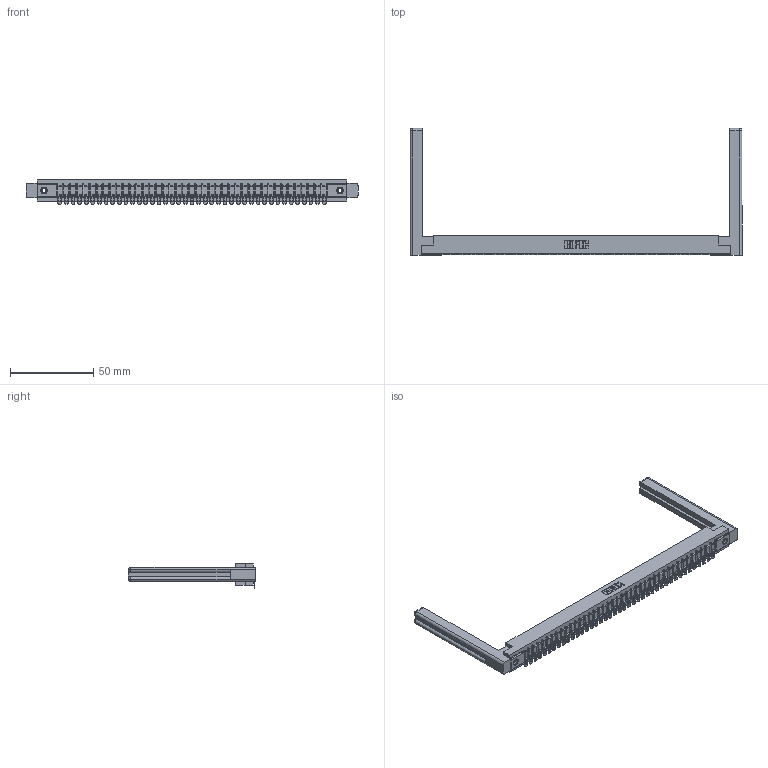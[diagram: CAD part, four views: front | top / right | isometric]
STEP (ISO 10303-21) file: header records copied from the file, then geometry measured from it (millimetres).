
FILE_DESCRIPTION (( 'STEP AP203' ), '1' );
FILE_NAME ('357-041-454-158.STEP', '2020-10-03T08:56:54', ( '' ), ( '' ), 'SwSTEP 2.0', 'SolidWorks 2020', '' );
FILE_SCHEMA (( 'CONFIG_CONTROL_DESIGN' ));
Length unit declared in the file: inch
Products named in the file (5): 345-250-001_345-250-001-102; 357-041-454-158; 307 Part_.156 Dia Mounting Holes; 307-290-002_554; 307-220-058
Assembly tree (46 placements, depth 2):
  357-041-454-158
    307 Part_.156 Dia Mounting Holes
    307-290-002_554  x41
    307-220-058  x2
    345-250-001_345-250-001-102  x2
Bounding box: 199.09 x 76.33 x 14.52 mm (x, y, z)
Volume: 28432.2 mm3; surface area: 31764.5 mm2
Topology: 46 solids, 46 shells, 3623 faces, 11050 edges, 7240 vertices
Faces by surface type: plane 2040, cylinder 1475, sphere 84, torus 12, cone 12
Entity records: 38870 total; most frequent: CARTESIAN_POINT 6565, ORIENTED_EDGE 6494, DIRECTION 6345, EDGE_CURVE 3247, LINE 2477, VECTOR 2477, VERTEX_POINT 2100, AXIS2_PLACEMENT_3D 1934
